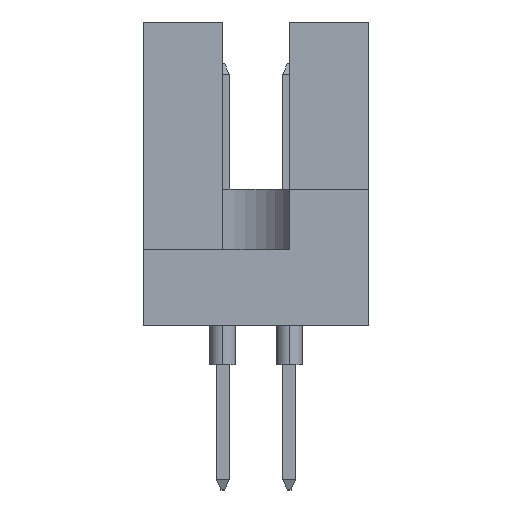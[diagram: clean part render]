
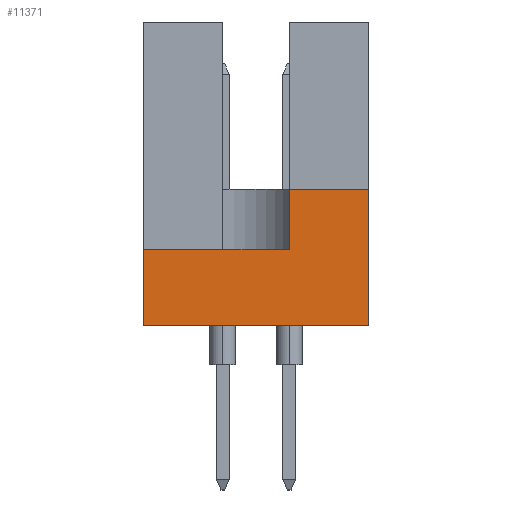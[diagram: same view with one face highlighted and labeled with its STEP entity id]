
A CAD part, left-side view. The second image highlights one B-rep face of the part: STEP entity #11371.
In plain terms, the highlighted planar face has unit normal (-1, 0, 0).
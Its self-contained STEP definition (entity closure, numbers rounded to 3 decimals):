
#55 = AXIS2_PLACEMENT_3D ( 'NONE', #2663, #5476, #9199 ) ;
#147 = LINE ( 'NONE', #11267, #6351 ) ;
#1295 = EDGE_CURVE ( 'NONE', #7953, #8501, #147, .T. ) ;
#1739 = CARTESIAN_POINT ( 'NONE',  ( -47.5, 4.3, 11.6 ) ) ;
#1863 = DIRECTION ( 'NONE',  ( 0., 0., -1. ) ) ;
#1965 = CARTESIAN_POINT ( 'NONE',  ( -47.5, 4.3, 0. ) ) ;
#2557 = VECTOR ( 'NONE', #10912, 1000. ) ;
#2595 = FACE_OUTER_BOUND ( 'NONE', #4420, .T. ) ;
#2663 = CARTESIAN_POINT ( 'NONE',  ( -47.5, 4.3, 11.6 ) ) ;
#2964 = VECTOR ( 'NONE', #3140, 1000. ) ;
#3140 = DIRECTION ( 'NONE',  ( 0., 0., -1. ) ) ;
#3683 = DIRECTION ( 'NONE',  ( 0., -1., 0. ) ) ;
#4176 = VECTOR ( 'NONE', #1863, 1000. ) ;
#4308 = CARTESIAN_POINT ( 'NONE',  ( -47.5, -1.27, 5.2 ) ) ;
#4326 = VECTOR ( 'NONE', #9995, 1000. ) ;
#4420 = EDGE_LOOP ( 'NONE', ( #9869, #11299, #9916, #11184, #10353, #7561 ) ) ;
#5476 = DIRECTION ( 'NONE',  ( 1., 0., 0. ) ) ;
#6151 = CARTESIAN_POINT ( 'NONE',  ( -47.5, -4.3, 11.6 ) ) ;
#6250 = EDGE_CURVE ( 'NONE', #11425, #9500, #7934, .T. ) ;
#6326 = LINE ( 'NONE', #6151, #2557 ) ;
#6351 = VECTOR ( 'NONE', #3683, 1000. ) ;
#6793 = CARTESIAN_POINT ( 'NONE',  ( -47.5, -4.3, 0. ) ) ;
#6928 = CARTESIAN_POINT ( 'NONE',  ( -47.5, -4.3, 5.2 ) ) ;
#7147 = LINE ( 'NONE', #9936, #4326 ) ;
#7561 = ORIENTED_EDGE ( 'NONE', *, *, #10285, .F. ) ;
#7934 = LINE ( 'NONE', #10718, #8119 ) ;
#7953 = VERTEX_POINT ( 'NONE', #1965 ) ;
#8119 = VECTOR ( 'NONE', #8664, 1000. ) ;
#8123 = CARTESIAN_POINT ( 'NONE',  ( -47.5, -1.27, 2.9 ) ) ;
#8501 = VERTEX_POINT ( 'NONE', #6793 ) ;
#8607 = LINE ( 'NONE', #8666, #2964 ) ;
#8664 = DIRECTION ( 'NONE',  ( 0., -1., 0. ) ) ;
#8666 = CARTESIAN_POINT ( 'NONE',  ( -47.5, -1.27, 19.02 ) ) ;
#8856 = CARTESIAN_POINT ( 'NONE',  ( -47.5, 4.3, 2.9 ) ) ;
#9022 = PLANE ( 'NONE',  #55 ) ;
#9144 = EDGE_CURVE ( 'NONE', #10377, #10814, #7147, .T. ) ;
#9199 = DIRECTION ( 'NONE',  ( 0., 0., -1. ) ) ;
#9267 = LINE ( 'NONE', #1739, #4176 ) ;
#9297 = EDGE_CURVE ( 'NONE', #10814, #7953, #9267, .T. ) ;
#9500 = VERTEX_POINT ( 'NONE', #6928 ) ;
#9869 = ORIENTED_EDGE ( 'NONE', *, *, #6250, .F. ) ;
#9916 = ORIENTED_EDGE ( 'NONE', *, *, #9144, .T. ) ;
#9936 = CARTESIAN_POINT ( 'NONE',  ( -47.5, 4.3, 2.9 ) ) ;
#9995 = DIRECTION ( 'NONE',  ( 0., 1., 0. ) ) ;
#10285 = EDGE_CURVE ( 'NONE', #9500, #8501, #6326, .T. ) ;
#10353 = ORIENTED_EDGE ( 'NONE', *, *, #1295, .T. ) ;
#10377 = VERTEX_POINT ( 'NONE', #8123 ) ;
#10718 = CARTESIAN_POINT ( 'NONE',  ( -47.5, 4.3, 5.2 ) ) ;
#10814 = VERTEX_POINT ( 'NONE', #8856 ) ;
#10912 = DIRECTION ( 'NONE',  ( 0., 0., -1. ) ) ;
#11184 = ORIENTED_EDGE ( 'NONE', *, *, #9297, .T. ) ;
#11267 = CARTESIAN_POINT ( 'NONE',  ( -47.5, 4.3, 0. ) ) ;
#11299 = ORIENTED_EDGE ( 'NONE', *, *, #11678, .T. ) ;
#11371 = ADVANCED_FACE ( 'NONE', ( #2595 ), #9022, .F. ) ;
#11425 = VERTEX_POINT ( 'NONE', #4308 ) ;
#11678 = EDGE_CURVE ( 'NONE', #11425, #10377, #8607, .T. ) ;
